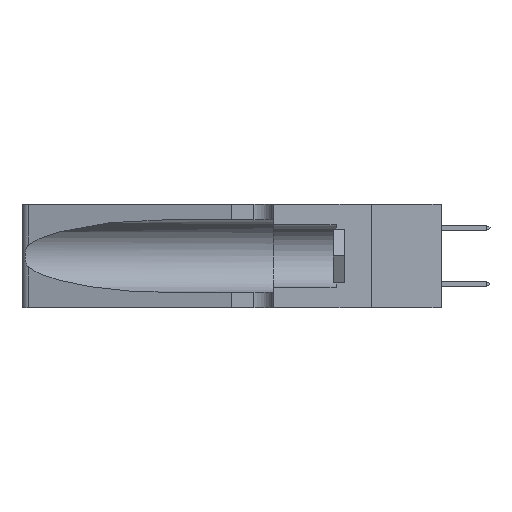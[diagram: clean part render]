
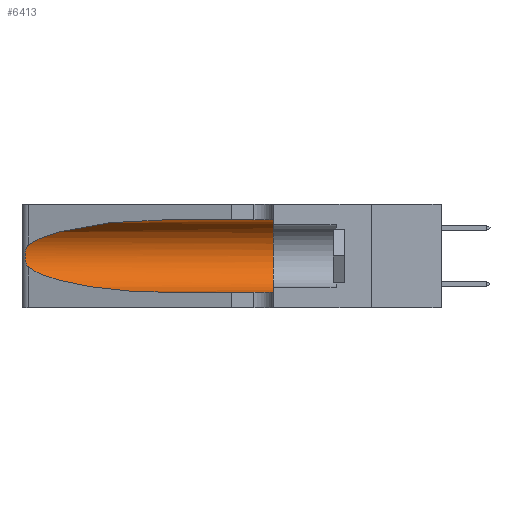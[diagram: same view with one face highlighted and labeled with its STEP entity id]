
A CAD part, left-side view. The second image highlights one B-rep face of the part: STEP entity #6413.
In plain terms, the highlighted cylindrical face has radius 3.308 mm (diameter 6.617 mm), a partial arc.
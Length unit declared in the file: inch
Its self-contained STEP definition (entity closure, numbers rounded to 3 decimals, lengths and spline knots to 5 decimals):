
#81 = CARTESIAN_POINT ( 'NONE',  ( 0.25487, 1.22718, 0.14631 ) ) ;
#324 = CARTESIAN_POINT ( 'NONE',  ( 0.26075, 1.23896, 0.19203 ) ) ;
#1528 = CARTESIAN_POINT ( 'NONE',  ( 0.25639, 1.23186, 0.15144 ) ) ;
#1753 = CARTESIAN_POINT ( 'NONE',  ( 0.1305, 1.61858, 0.31525 ) ) ;
#2027 = CARTESIAN_POINT ( 'NONE',  ( 0.1305, 0.72297, 0.31525 ) ) ;
#2901 = EDGE_CURVE ( 'NONE', #9832, #10937, #6429, .T. ) ;
#2945 = DIRECTION ( 'NONE',  ( 0., -1., 0. ) ) ;
#3078 = CARTESIAN_POINT ( 'NONE',  ( 0.25639, 1.23184, 0.21858 ) ) ;
#3092 = ORIENTED_EDGE ( 'NONE', *, *, #10213, .T. ) ;
#3097 = CARTESIAN_POINT ( 'NONE',  ( 0.25487, 1.22718, 0.14631 ) ) ;
#3306 = CARTESIAN_POINT ( 'NONE',  ( 0.1305, 1.61858, 0.185 ) ) ;
#3430 = DIRECTION ( 'NONE',  ( 0., 0., -1. ) ) ;
#4014 = ORIENTED_EDGE ( 'NONE', *, *, #16173, .F. ) ;
#4451 = CARTESIAN_POINT ( 'NONE',  ( 0.25856, 1.23593, 0.16098 ) ) ;
#4509 = CARTESIAN_POINT ( 'NONE',  ( 0.26075, 1.23896, 0.178 ) ) ;
#5046 = VERTEX_POINT ( 'NONE', #12881 ) ;
#5438 = EDGE_CURVE ( 'NONE', #16791, #5046, #13703, .T. ) ;
#5707 = VECTOR ( 'NONE', #5778, 39.37008 ) ;
#5778 = DIRECTION ( 'NONE',  ( 0., -1., 0. ) ) ;
#5789 = ORIENTED_EDGE ( 'NONE', *, *, #9843, .T. ) ;
#6413 = ADVANCED_FACE ( 'NONE', ( #8513 ), #9383, .F. ) ;
#6429 = CIRCLE ( 'NONE', #14588, 0.13025 ) ;
#6657 = EDGE_LOOP ( 'NONE', ( #5789, #3092, #8438, #17910, #10167, #4014 ) ) ;
#6835 = VERTEX_POINT ( 'NONE', #11460 ) ;
#7223 = CARTESIAN_POINT ( 'NONE',  ( 0.25555, 1.22994, 0.2215 ) ) ;
#7254 = CARTESIAN_POINT ( 'NONE',  ( 0.25487, 1.22718, 0.22369 ) ) ;
#7385 = CARTESIAN_POINT ( 'NONE',  ( 0.25487, 1.22718, 0.14631 ) ) ;
#8026 = CARTESIAN_POINT ( 'NONE',  ( 0.1305, 0.35, 0.185 ) ) ;
#8039 = AXIS2_PLACEMENT_3D ( 'NONE', #3306, #13202, #3430 ) ;
#8438 = ORIENTED_EDGE ( 'NONE', *, *, #5438, .T. ) ;
#8513 = FACE_OUTER_BOUND ( 'NONE', #6657, .T. ) ;
#8624 = CARTESIAN_POINT ( 'NONE',  ( 0.25487, 1.22718, 0.22369 ) ) ;
#8795 = CARTESIAN_POINT ( 'NONE',  ( 0.25854, 1.2359, 0.20912 ) ) ;
#9174 = CARTESIAN_POINT ( 'NONE',  ( 0.1305, 0.35, 0.31525 ) ) ;
#9371 = CARTESIAN_POINT ( 'NONE',  ( 0.25487, 1.22718, 0.22369 ) ) ;
#9383 = CYLINDRICAL_SURFACE ( 'NONE', #8039, 0.13025 ) ;
#9832 = VERTEX_POINT ( 'NONE', #9174 ) ;
#9843 = EDGE_CURVE ( 'NONE', #6835, #13507, #10405, .T. ) ;
#9956 = CARTESIAN_POINT ( 'NONE',  ( 0.18966, 0.96281, 0.05475 ) ) ;
#10131 = CARTESIAN_POINT ( 'NONE',  ( 0.26018, 1.23835, 0.19895 ) ) ;
#10167 = ORIENTED_EDGE ( 'NONE', *, *, #2901, .F. ) ;
#10187 = EDGE_CURVE ( 'NONE', #5046, #10937, #16021, .T. ) ;
#10213 = EDGE_CURVE ( 'NONE', #13507, #16791, #15047, .T. ) ;
#10405 =( BOUNDED_CURVE ( )  B_SPLINE_CURVE ( 3, ( #2027, #11940, #17743, #9371 ),
 .UNSPECIFIED., .F., .F. ) 
 B_SPLINE_CURVE_WITH_KNOTS ( ( 4, 4 ),
 ( 1.5708, 2.84003 ),
 .UNSPECIFIED. ) 
 CURVE ( )  GEOMETRIC_REPRESENTATION_ITEM ( )  RATIONAL_B_SPLINE_CURVE ( ( 1., 0.87, 0.87, 1. ) ) 
 REPRESENTATION_ITEM ( '' )  );
#10800 = DIRECTION ( 'NONE',  ( 0., 1., 0. ) ) ;
#10937 = VERTEX_POINT ( 'NONE', #17381 ) ;
#11443 = CARTESIAN_POINT ( 'NONE',  ( 0.25789, 1.23486, 0.15765 ) ) ;
#11460 = CARTESIAN_POINT ( 'NONE',  ( 0.1305, 0.72297, 0.31525 ) ) ;
#11503 = VECTOR ( 'NONE', #2945, 39.37008 ) ;
#11940 = CARTESIAN_POINT ( 'NONE',  ( 0.18966, 0.96281, 0.31525 ) ) ;
#12408 = DIRECTION ( 'NONE',  ( 0., 0., 1. ) ) ;
#12616 = CARTESIAN_POINT ( 'NONE',  ( 0.2373, 1.15595, 0.08982 ) ) ;
#12881 = CARTESIAN_POINT ( 'NONE',  ( 0.1305, 0.72297, 0.05475 ) ) ;
#13202 = DIRECTION ( 'NONE',  ( 0., -1., 0. ) ) ;
#13507 = VERTEX_POINT ( 'NONE', #7254 ) ;
#13703 =( BOUNDED_CURVE ( )  B_SPLINE_CURVE ( 3, ( #81, #12616, #9956, #14077 ),
 .UNSPECIFIED., .F., .T. ) 
 B_SPLINE_CURVE_WITH_KNOTS ( ( 4, 4 ),
 ( 3.44316, 4.71239 ),
 .UNSPECIFIED. ) 
 CURVE ( )  GEOMETRIC_REPRESENTATION_ITEM ( )  RATIONAL_B_SPLINE_CURVE ( ( 1., 0.87, 0.87, 1. ) ) 
 REPRESENTATION_ITEM ( '' )  );
#14077 = CARTESIAN_POINT ( 'NONE',  ( 0.1305, 0.72297, 0.05475 ) ) ;
#14263 = CARTESIAN_POINT ( 'NONE',  ( 0.1305, 1.61858, 0.05475 ) ) ;
#14588 = AXIS2_PLACEMENT_3D ( 'NONE', #8026, #10800, #12408 ) ;
#15047 = B_SPLINE_CURVE_WITH_KNOTS ( 'NONE', 3,
 ( #8624, #7223, #3078, #17223, #8795, #10131, #324, #4509, #17050, #4451, #11443, #1528, #15842, #7385 ),
 .UNSPECIFIED., .F., .F.,
 ( 4, 2, 2, 2, 2, 2, 4 ),
 ( 0., 0.00027, 0.00053, 0.00107, 0.0016, 0.00187, 0.00214 ),
 .UNSPECIFIED. ) ;
#15842 = CARTESIAN_POINT ( 'NONE',  ( 0.25555, 1.22993, 0.14849 ) ) ;
#16021 = LINE ( 'NONE', #14263, #5707 ) ;
#16173 = EDGE_CURVE ( 'NONE', #6835, #9832, #16800, .T. ) ;
#16791 = VERTEX_POINT ( 'NONE', #3097 ) ;
#16800 = LINE ( 'NONE', #1753, #11503 ) ;
#17050 = CARTESIAN_POINT ( 'NONE',  ( 0.26017, 1.23833, 0.17102 ) ) ;
#17223 = CARTESIAN_POINT ( 'NONE',  ( 0.25787, 1.23484, 0.2124 ) ) ;
#17381 = CARTESIAN_POINT ( 'NONE',  ( 0.1305, 0.35, 0.05475 ) ) ;
#17743 = CARTESIAN_POINT ( 'NONE',  ( 0.2373, 1.15595, 0.28018 ) ) ;
#17910 = ORIENTED_EDGE ( 'NONE', *, *, #10187, .T. ) ;
